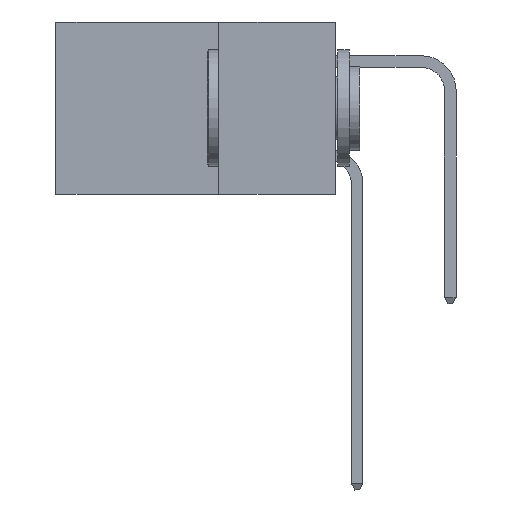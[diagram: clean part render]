
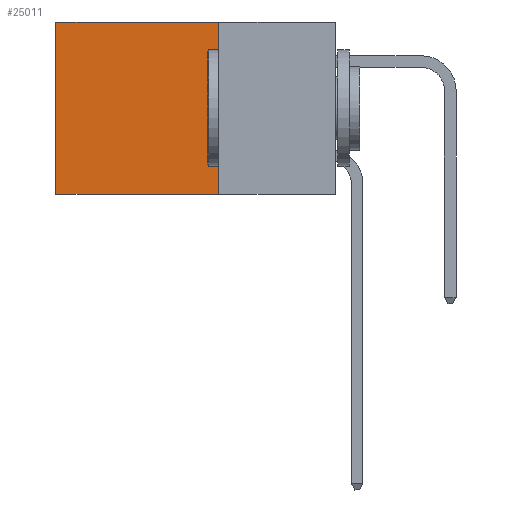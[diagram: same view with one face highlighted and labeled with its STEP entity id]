
A CAD part, left-side view. The second image highlights one B-rep face of the part: STEP entity #25011.
In plain terms, the highlighted planar face has unit normal (-1, 0, 0).
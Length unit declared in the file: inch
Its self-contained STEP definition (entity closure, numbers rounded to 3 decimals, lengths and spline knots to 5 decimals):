
#330 = VECTOR ( 'NONE', #14694, 39.37008 ) ;
#686 = ORIENTED_EDGE ( 'NONE', *, *, #12263, .T. ) ;
#1015 = LINE ( 'NONE', #27288, #330 ) ;
#3217 = PLANE ( 'NONE',  #22094 ) ;
#3300 = CARTESIAN_POINT ( 'NONE',  ( 0.2875, 0.25, 0. ) ) ;
#3332 = VERTEX_POINT ( 'NONE', #20101 ) ;
#5491 = DIRECTION ( 'NONE',  ( 0., 0., -1. ) ) ;
#6315 = ORIENTED_EDGE ( 'NONE', *, *, #16809, .T. ) ;
#6503 = LINE ( 'NONE', #10097, #17112 ) ;
#7072 = VERTEX_POINT ( 'NONE', #24185 ) ;
#7399 = LINE ( 'NONE', #23498, #22871 ) ;
#10081 = CARTESIAN_POINT ( 'NONE',  ( 0.2875, 0.6, 0. ) ) ;
#10097 = CARTESIAN_POINT ( 'NONE',  ( 0.2875, 0.25, 0. ) ) ;
#10674 = ORIENTED_EDGE ( 'NONE', *, *, #19448, .F. ) ;
#11379 = FACE_OUTER_BOUND ( 'NONE', #21568, .T. ) ;
#12263 = EDGE_CURVE ( 'NONE', #7072, #3332, #26348, .T. ) ;
#12389 = VERTEX_POINT ( 'NONE', #23086 ) ;
#13383 = VERTEX_POINT ( 'NONE', #13554 ) ;
#13554 = CARTESIAN_POINT ( 'NONE',  ( 0.2875, 0.25, 0. ) ) ;
#14694 = DIRECTION ( 'NONE',  ( 0., 0., -1. ) ) ;
#16809 = EDGE_CURVE ( 'NONE', #13383, #7072, #6503, .T. ) ;
#17112 = VECTOR ( 'NONE', #22542, 39.37008 ) ;
#18164 = DIRECTION ( 'NONE',  ( 1., 0., 0. ) ) ;
#19350 = DIRECTION ( 'NONE',  ( 0., 1., 0. ) ) ;
#19448 = EDGE_CURVE ( 'NONE', #12389, #3332, #7399, .T. ) ;
#20101 = CARTESIAN_POINT ( 'NONE',  ( 0.2875, 0.6, -0.37 ) ) ;
#20758 = VECTOR ( 'NONE', #26900, 39.37008 ) ;
#21568 = EDGE_LOOP ( 'NONE', ( #686, #10674, #25281, #6315 ) ) ;
#22094 = AXIS2_PLACEMENT_3D ( 'NONE', #3300, #18164, #5491 ) ;
#22542 = DIRECTION ( 'NONE',  ( 0., 1., 0. ) ) ;
#22871 = VECTOR ( 'NONE', #19350, 39.37008 ) ;
#23086 = CARTESIAN_POINT ( 'NONE',  ( 0.2875, 0.25, -0.37 ) ) ;
#23498 = CARTESIAN_POINT ( 'NONE',  ( 0.2875, 0.25, -0.37 ) ) ;
#24185 = CARTESIAN_POINT ( 'NONE',  ( 0.2875, 0.6, 0. ) ) ;
#25011 = ADVANCED_FACE ( 'NONE', ( #11379 ), #3217, .F. ) ;
#25281 = ORIENTED_EDGE ( 'NONE', *, *, #27449, .F. ) ;
#26348 = LINE ( 'NONE', #10081, #20758 ) ;
#26900 = DIRECTION ( 'NONE',  ( 0., 0., -1. ) ) ;
#27288 = CARTESIAN_POINT ( 'NONE',  ( 0.2875, 0.25, 0. ) ) ;
#27449 = EDGE_CURVE ( 'NONE', #13383, #12389, #1015, .T. ) ;
